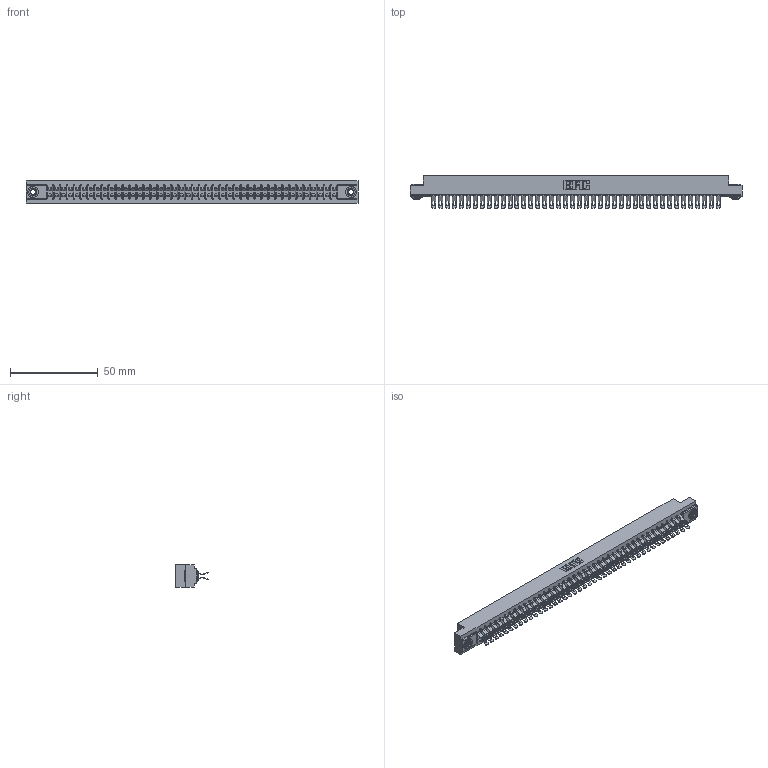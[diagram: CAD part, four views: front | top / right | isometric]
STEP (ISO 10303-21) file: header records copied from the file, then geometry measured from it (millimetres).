
FILE_DESCRIPTION (( 'STEP AP203' ), '1' );
FILE_NAME ('307-084-555-203.STEP', '2019-09-07T01:58:17', ( '' ), ( '' ), 'SwSTEP 2.0', 'SolidWorks 2016', '' );
FILE_SCHEMA (( 'CONFIG_CONTROL_DESIGN' ));
Length unit declared in the file: inch
Products named in the file (4): 345-250-002_345-250-002-102; 307-084-555-203; 307 Part_.156 Dia Mounting Holes; 307-290-001_555
Assembly tree (87 placements, depth 2):
  307-084-555-203
    307 Part_.156 Dia Mounting Holes
    307-290-001_555  x84
    345-250-002_345-250-002-102  x2
Bounding box: 189.43 x 18.75 x 12.7 mm (x, y, z)
Volume: 20395.6 mm3; surface area: 26594.7 mm2
Topology: 87 solids, 87 shells, 5337 faces, 15639 edges, 10194 vertices
Faces by surface type: plane 2950, cylinder 2293, sphere 86, cone 8
Entity records: 38952 total; most frequent: CARTESIAN_POINT 6359, ORIENTED_EDGE 6296, DIRECTION 6250, EDGE_CURVE 3148, LINE 2396, VECTOR 2396, VERTEX_POINT 2036, AXIS2_PLACEMENT_3D 1927
